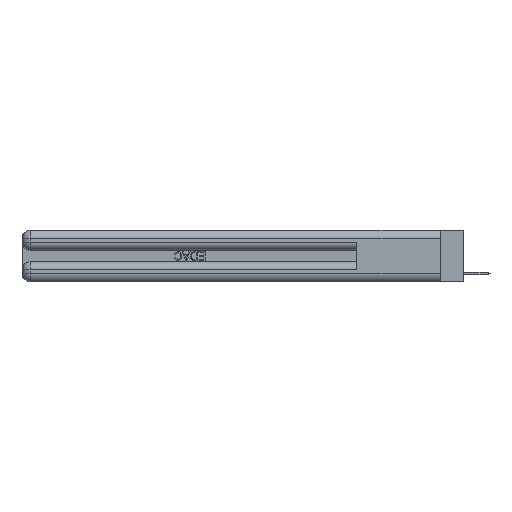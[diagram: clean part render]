
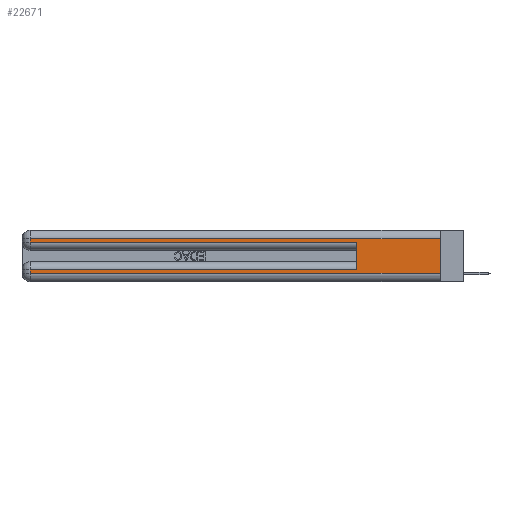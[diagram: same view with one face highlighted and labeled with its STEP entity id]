
A CAD part, left-side view. The second image highlights one B-rep face of the part: STEP entity #22671.
In plain terms, the highlighted planar face has unit normal (-1, 0, 0).
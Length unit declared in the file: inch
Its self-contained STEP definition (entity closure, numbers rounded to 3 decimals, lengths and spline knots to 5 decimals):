
#362 = DIRECTION ( 'NONE',  ( 0., -1., 0. ) ) ;
#440 = LINE ( 'NONE', #18795, #17697 ) ;
#454 = FACE_OUTER_BOUND ( 'NONE', #11640, .T. ) ;
#763 = VECTOR ( 'NONE', #9988, 39.37008 ) ;
#2037 = VERTEX_POINT ( 'NONE', #6439 ) ;
#2179 = ORIENTED_EDGE ( 'NONE', *, *, #31249, .T. ) ;
#2577 = AXIS2_PLACEMENT_3D ( 'NONE', #24104, #29949, #21531 ) ;
#3293 = VERTEX_POINT ( 'NONE', #5045 ) ;
#4058 = VECTOR ( 'NONE', #11169, 39.37008 ) ;
#4633 = ORIENTED_EDGE ( 'NONE', *, *, #17119, .T. ) ;
#4818 = CARTESIAN_POINT ( 'NONE',  ( 0., 0., 0.31 ) ) ;
#5045 = CARTESIAN_POINT ( 'NONE',  ( 0., 0., 0.06 ) ) ;
#5241 = DIRECTION ( 'NONE',  ( 0., 0., 1. ) ) ;
#5348 = EDGE_CURVE ( 'NONE', #33760, #2037, #26005, .T. ) ;
#5453 = VERTEX_POINT ( 'NONE', #13831 ) ;
#5742 = DIRECTION ( 'NONE',  ( 0., 0., -1. ) ) ;
#6439 = CARTESIAN_POINT ( 'NONE',  ( 0., 0.6, 0.285 ) ) ;
#6535 = ORIENTED_EDGE ( 'NONE', *, *, #12866, .T. ) ;
#6645 = CARTESIAN_POINT ( 'NONE',  ( 0., 2.94, 0.285 ) ) ;
#8048 = ORIENTED_EDGE ( 'NONE', *, *, #5348, .F. ) ;
#8675 = ORIENTED_EDGE ( 'NONE', *, *, #31327, .T. ) ;
#8932 = CARTESIAN_POINT ( 'NONE',  ( 0., 0., 0.37 ) ) ;
#9988 = DIRECTION ( 'NONE',  ( 0., 1., 0. ) ) ;
#11169 = DIRECTION ( 'NONE',  ( 0., 1., 0. ) ) ;
#11640 = EDGE_LOOP ( 'NONE', ( #29400, #4633, #21370, #2179, #8048, #8675, #16106, #6535 ) ) ;
#12357 = VECTOR ( 'NONE', #5241, 39.37008 ) ;
#12681 = VERTEX_POINT ( 'NONE', #30390 ) ;
#12866 = EDGE_CURVE ( 'NONE', #31786, #3293, #32906, .T. ) ;
#13831 = CARTESIAN_POINT ( 'NONE',  ( 0., 2.94, 0.085 ) ) ;
#13910 = LINE ( 'NONE', #8932, #23159 ) ;
#14970 = CARTESIAN_POINT ( 'NONE',  ( 0., 0., 0.285 ) ) ;
#15638 = CARTESIAN_POINT ( 'NONE',  ( 0., 0., 0.31 ) ) ;
#15932 = EDGE_CURVE ( 'NONE', #27706, #3293, #13910, .T. ) ;
#16106 = ORIENTED_EDGE ( 'NONE', *, *, #30505, .T. ) ;
#16995 = DIRECTION ( 'NONE',  ( 0., -1., 0. ) ) ;
#17002 = VECTOR ( 'NONE', #16995, 39.37008 ) ;
#17119 = EDGE_CURVE ( 'NONE', #27706, #12681, #33624, .T. ) ;
#17550 = LINE ( 'NONE', #14970, #27074 ) ;
#17697 = VECTOR ( 'NONE', #5742, 39.37008 ) ;
#18795 = CARTESIAN_POINT ( 'NONE',  ( 0., 2.94, 0.37 ) ) ;
#19377 = CARTESIAN_POINT ( 'NONE',  ( 0., 0., 0.06 ) ) ;
#21217 = VERTEX_POINT ( 'NONE', #6645 ) ;
#21370 = ORIENTED_EDGE ( 'NONE', *, *, #25998, .T. ) ;
#21531 = DIRECTION ( 'NONE',  ( 0., 0., -1. ) ) ;
#21780 = LINE ( 'NONE', #32239, #4058 ) ;
#22671 = ADVANCED_FACE ( 'NONE', ( #454 ), #27194, .F. ) ;
#22705 = CARTESIAN_POINT ( 'NONE',  ( 0., 2.94, 0.06 ) ) ;
#23159 = VECTOR ( 'NONE', #24344, 39.37008 ) ;
#23865 = CARTESIAN_POINT ( 'NONE',  ( 0., 0.6, 0.085 ) ) ;
#24104 = CARTESIAN_POINT ( 'NONE',  ( 0., 0., 0.37 ) ) ;
#24344 = DIRECTION ( 'NONE',  ( 0., 0., -1. ) ) ;
#25998 = EDGE_CURVE ( 'NONE', #12681, #21217, #33648, .T. ) ;
#26005 = LINE ( 'NONE', #28750, #12357 ) ;
#27074 = VECTOR ( 'NONE', #362, 39.37008 ) ;
#27194 = PLANE ( 'NONE',  #2577 ) ;
#27706 = VERTEX_POINT ( 'NONE', #4818 ) ;
#28750 = CARTESIAN_POINT ( 'NONE',  ( 0., 0.6, 0.145 ) ) ;
#29028 = DIRECTION ( 'NONE',  ( 0., 0., -1. ) ) ;
#29400 = ORIENTED_EDGE ( 'NONE', *, *, #15932, .F. ) ;
#29582 = VECTOR ( 'NONE', #29028, 39.37008 ) ;
#29949 = DIRECTION ( 'NONE',  ( 1., 0., 0. ) ) ;
#30390 = CARTESIAN_POINT ( 'NONE',  ( 0., 2.94, 0.31 ) ) ;
#30505 = EDGE_CURVE ( 'NONE', #5453, #31786, #440, .T. ) ;
#31249 = EDGE_CURVE ( 'NONE', #21217, #2037, #17550, .T. ) ;
#31327 = EDGE_CURVE ( 'NONE', #33760, #5453, #21780, .T. ) ;
#31786 = VERTEX_POINT ( 'NONE', #22705 ) ;
#32239 = CARTESIAN_POINT ( 'NONE',  ( 0., 0., 0.085 ) ) ;
#32906 = LINE ( 'NONE', #19377, #17002 ) ;
#33312 = CARTESIAN_POINT ( 'NONE',  ( 0., 2.94, 0.37 ) ) ;
#33624 = LINE ( 'NONE', #15638, #763 ) ;
#33648 = LINE ( 'NONE', #33312, #29582 ) ;
#33760 = VERTEX_POINT ( 'NONE', #23865 ) ;
